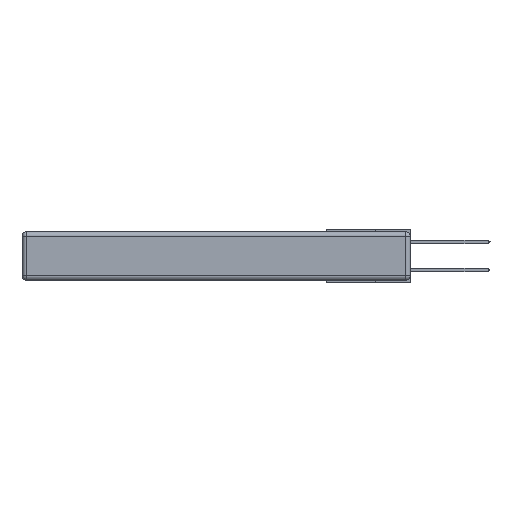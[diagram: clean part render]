
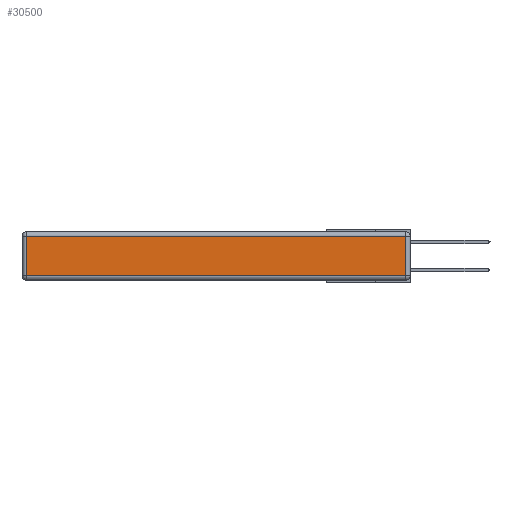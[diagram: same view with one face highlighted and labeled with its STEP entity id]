
A CAD part, left-side view. The second image highlights one B-rep face of the part: STEP entity #30500.
In plain terms, the highlighted planar face has unit normal (-1, 0, 0).
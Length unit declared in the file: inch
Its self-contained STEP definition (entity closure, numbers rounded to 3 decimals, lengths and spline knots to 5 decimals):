
#398 = CARTESIAN_POINT ( 'NONE',  ( 0., 2.75, -0.03 ) ) ;
#1059 = LINE ( 'NONE', #398, #4720 ) ;
#1710 = VERTEX_POINT ( 'NONE', #3355 ) ;
#2158 = CARTESIAN_POINT ( 'NONE',  ( 0., 0.03, -0.343 ) ) ;
#2189 = CARTESIAN_POINT ( 'NONE',  ( 0., 0.03, -0.03 ) ) ;
#3355 = CARTESIAN_POINT ( 'NONE',  ( 0., 2.72, -0.03 ) ) ;
#4720 = VECTOR ( 'NONE', #26433, 39.37008 ) ;
#5219 = FACE_OUTER_BOUND ( 'NONE', #15900, .T. ) ;
#6921 = DIRECTION ( 'NONE',  ( 0., 0., 1. ) ) ;
#8446 = ORIENTED_EDGE ( 'NONE', *, *, #21118, .T. ) ;
#9149 = CARTESIAN_POINT ( 'NONE',  ( 0., 0., -0.313 ) ) ;
#10303 = ORIENTED_EDGE ( 'NONE', *, *, #22752, .T. ) ;
#10753 = CARTESIAN_POINT ( 'NONE',  ( 0., 0.03, -0.313 ) ) ;
#11073 = VECTOR ( 'NONE', #12932, 39.37008 ) ;
#11537 = VECTOR ( 'NONE', #6921, 39.37008 ) ;
#12932 = DIRECTION ( 'NONE',  ( 0., 0., -1. ) ) ;
#13765 = LINE ( 'NONE', #2158, #11537 ) ;
#14146 = CARTESIAN_POINT ( 'NONE',  ( 0., 0., -0.343 ) ) ;
#15199 = LINE ( 'NONE', #15351, #11073 ) ;
#15351 = CARTESIAN_POINT ( 'NONE',  ( 0., 2.72, -0.343 ) ) ;
#15900 = EDGE_LOOP ( 'NONE', ( #10303, #27278, #21920, #8446 ) ) ;
#16374 = EDGE_CURVE ( 'NONE', #23299, #28188, #13765, .T. ) ;
#18257 = AXIS2_PLACEMENT_3D ( 'NONE', #14146, #30408, #30829 ) ;
#19918 = CARTESIAN_POINT ( 'NONE',  ( 0., 2.72, -0.313 ) ) ;
#21118 = EDGE_CURVE ( 'NONE', #1710, #23744, #15199, .T. ) ;
#21920 = ORIENTED_EDGE ( 'NONE', *, *, #26041, .T. ) ;
#22752 = EDGE_CURVE ( 'NONE', #23744, #23299, #25492, .T. ) ;
#23259 = DIRECTION ( 'NONE',  ( 0., -1., 0. ) ) ;
#23299 = VERTEX_POINT ( 'NONE', #10753 ) ;
#23744 = VERTEX_POINT ( 'NONE', #19918 ) ;
#25492 = LINE ( 'NONE', #9149, #27011 ) ;
#26041 = EDGE_CURVE ( 'NONE', #28188, #1710, #1059, .T. ) ;
#26433 = DIRECTION ( 'NONE',  ( 0., 1., 0. ) ) ;
#27011 = VECTOR ( 'NONE', #23259, 39.37008 ) ;
#27278 = ORIENTED_EDGE ( 'NONE', *, *, #16374, .T. ) ;
#28188 = VERTEX_POINT ( 'NONE', #2189 ) ;
#30408 = DIRECTION ( 'NONE',  ( -1., 0., 0. ) ) ;
#30500 = ADVANCED_FACE ( 'NONE', ( #5219 ), #30513, .T. ) ;
#30513 = PLANE ( 'NONE',  #18257 ) ;
#30829 = DIRECTION ( 'NONE',  ( 0., 0., 1. ) ) ;
